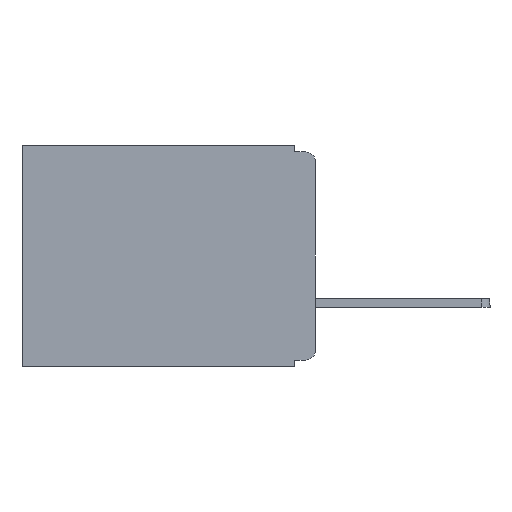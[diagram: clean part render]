
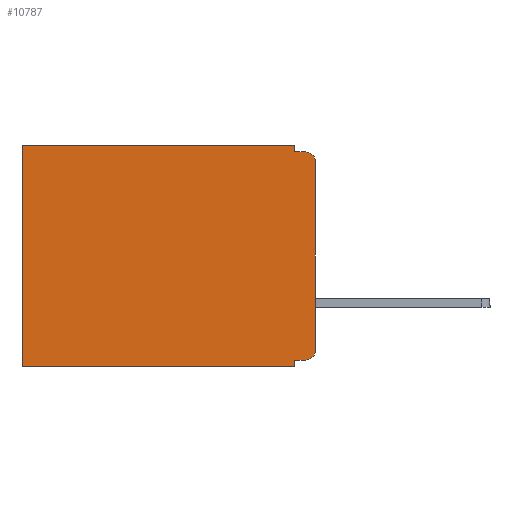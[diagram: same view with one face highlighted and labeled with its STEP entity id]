
A CAD part, left-side view. The second image highlights one B-rep face of the part: STEP entity #10787.
In plain terms, the highlighted planar face has unit normal (-1, 0, 0).
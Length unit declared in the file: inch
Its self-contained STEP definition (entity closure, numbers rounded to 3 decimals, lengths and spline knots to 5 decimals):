
#88 = LINE ( 'NONE', #7431, #16410 ) ;
#299 = CIRCLE ( 'NONE', #828, 0.015 ) ;
#390 = DIRECTION ( 'NONE',  ( 0., 0., -1. ) ) ;
#621 = EDGE_CURVE ( 'NONE', #9456, #8271, #6126, .T. ) ;
#828 = AXIS2_PLACEMENT_3D ( 'NONE', #17038, #7433, #18661 ) ;
#851 = EDGE_CURVE ( 'NONE', #11710, #12561, #5374, .T. ) ;
#950 = DIRECTION ( 'NONE',  ( 0., -1., 0. ) ) ;
#1039 = LINE ( 'NONE', #16659, #19556 ) ;
#1273 = CARTESIAN_POINT ( 'NONE',  ( 0.3, 0.031, -0.33 ) ) ;
#1538 = CIRCLE ( 'NONE', #13195, 0.015 ) ;
#1649 = EDGE_CURVE ( 'NONE', #15379, #8201, #2209, .T. ) ;
#2209 = LINE ( 'NONE', #11035, #15659 ) ;
#2233 = DIRECTION ( 'NONE',  ( 0., 0., -1. ) ) ;
#2253 = VECTOR ( 'NONE', #6494, 39.37008 ) ;
#2718 = CARTESIAN_POINT ( 'NONE',  ( 0.3, 0., -0.305 ) ) ;
#3698 = CARTESIAN_POINT ( 'NONE',  ( 0.3, 0.031, 0. ) ) ;
#3895 = ORIENTED_EDGE ( 'NONE', *, *, #20983, .F. ) ;
#4045 = ORIENTED_EDGE ( 'NONE', *, *, #851, .F. ) ;
#4522 = CARTESIAN_POINT ( 'NONE',  ( 0.3, 0., -0.33 ) ) ;
#4818 = CARTESIAN_POINT ( 'NONE',  ( 0.3, 0.015, -0.305 ) ) ;
#4846 = ORIENTED_EDGE ( 'NONE', *, *, #1649, .T. ) ;
#5374 = LINE ( 'NONE', #1273, #17690 ) ;
#5652 = LINE ( 'NONE', #4522, #13681 ) ;
#6126 = LINE ( 'NONE', #18607, #14677 ) ;
#6450 = EDGE_CURVE ( 'NONE', #10704, #15379, #88, .T. ) ;
#6462 = DIRECTION ( 'NONE',  ( 0., 0., -1. ) ) ;
#6494 = DIRECTION ( 'NONE',  ( 0., 1., 0. ) ) ;
#6562 = CARTESIAN_POINT ( 'NONE',  ( 0.3, 0., -0.32 ) ) ;
#7431 = CARTESIAN_POINT ( 'NONE',  ( 0.3, 0., 0. ) ) ;
#7433 = DIRECTION ( 'NONE',  ( -1., 0., 0. ) ) ;
#8042 = VERTEX_POINT ( 'NONE', #19347 ) ;
#8201 = VERTEX_POINT ( 'NONE', #16296 ) ;
#8271 = VERTEX_POINT ( 'NONE', #10420 ) ;
#8680 = EDGE_CURVE ( 'NONE', #20669, #17223, #1538, .T. ) ;
#8954 = ORIENTED_EDGE ( 'NONE', *, *, #20489, .F. ) ;
#9442 = DIRECTION ( 'NONE',  ( 0., 0., -1. ) ) ;
#9456 = VERTEX_POINT ( 'NONE', #11789 ) ;
#9977 = DIRECTION ( 'NONE',  ( 0., 0., -1. ) ) ;
#10138 = EDGE_CURVE ( 'NONE', #12561, #8201, #1039, .T. ) ;
#10391 = CARTESIAN_POINT ( 'NONE',  ( 0.3, 0., -0.33 ) ) ;
#10420 = CARTESIAN_POINT ( 'NONE',  ( 0.3, 0.015, -0.01 ) ) ;
#10456 = LINE ( 'NONE', #6562, #2253 ) ;
#10574 = CARTESIAN_POINT ( 'NONE',  ( 0.3, 0.437, 0. ) ) ;
#10639 = EDGE_CURVE ( 'NONE', #10704, #9456, #19055, .T. ) ;
#10704 = VERTEX_POINT ( 'NONE', #3698 ) ;
#10787 = ADVANCED_FACE ( 'NONE', ( #15529 ), #19952, .F. ) ;
#11035 = CARTESIAN_POINT ( 'NONE',  ( 0.3, 0.437, -0.33 ) ) ;
#11106 = DIRECTION ( 'NONE',  ( 0., 0., -1. ) ) ;
#11425 = DIRECTION ( 'NONE',  ( 0., 1., 0. ) ) ;
#11710 = VERTEX_POINT ( 'NONE', #20813 ) ;
#11789 = CARTESIAN_POINT ( 'NONE',  ( 0.3, 0.031, -0.01 ) ) ;
#12016 = DIRECTION ( 'NONE',  ( 1., 0., 0. ) ) ;
#12436 = AXIS2_PLACEMENT_3D ( 'NONE', #10391, #12016, #2233 ) ;
#12561 = VERTEX_POINT ( 'NONE', #19966 ) ;
#12746 = ORIENTED_EDGE ( 'NONE', *, *, #10639, .F. ) ;
#13195 = AXIS2_PLACEMENT_3D ( 'NONE', #4818, #16075, #6462 ) ;
#13681 = VECTOR ( 'NONE', #9442, 39.37008 ) ;
#14677 = VECTOR ( 'NONE', #950, 39.37008 ) ;
#14786 = EDGE_CURVE ( 'NONE', #8042, #8271, #299, .T. ) ;
#14794 = VECTOR ( 'NONE', #9977, 39.37008 ) ;
#14969 = CARTESIAN_POINT ( 'NONE',  ( 0.3, 0.015, -0.32 ) ) ;
#15168 = ORIENTED_EDGE ( 'NONE', *, *, #10138, .F. ) ;
#15379 = VERTEX_POINT ( 'NONE', #10574 ) ;
#15427 = ORIENTED_EDGE ( 'NONE', *, *, #6450, .T. ) ;
#15529 = FACE_OUTER_BOUND ( 'NONE', #20500, .T. ) ;
#15659 = VECTOR ( 'NONE', #390, 39.37008 ) ;
#16075 = DIRECTION ( 'NONE',  ( -1., 0., 0. ) ) ;
#16296 = CARTESIAN_POINT ( 'NONE',  ( 0.3, 0.437, -0.33 ) ) ;
#16410 = VECTOR ( 'NONE', #11425, 39.37008 ) ;
#16583 = DIRECTION ( 'NONE',  ( 0., 1., 0. ) ) ;
#16659 = CARTESIAN_POINT ( 'NONE',  ( 0.3, 0., -0.33 ) ) ;
#17038 = CARTESIAN_POINT ( 'NONE',  ( 0.3, 0.015, -0.025 ) ) ;
#17223 = VERTEX_POINT ( 'NONE', #2718 ) ;
#17690 = VECTOR ( 'NONE', #11106, 39.37008 ) ;
#17968 = ORIENTED_EDGE ( 'NONE', *, *, #621, .F. ) ;
#18572 = ORIENTED_EDGE ( 'NONE', *, *, #8680, .T. ) ;
#18607 = CARTESIAN_POINT ( 'NONE',  ( 0.3, 0., -0.01 ) ) ;
#18661 = DIRECTION ( 'NONE',  ( 0., 0., -1. ) ) ;
#19055 = LINE ( 'NONE', #19552, #14794 ) ;
#19347 = CARTESIAN_POINT ( 'NONE',  ( 0.3, 0., -0.025 ) ) ;
#19552 = CARTESIAN_POINT ( 'NONE',  ( 0.3, 0.031, 0. ) ) ;
#19556 = VECTOR ( 'NONE', #16583, 39.37008 ) ;
#19952 = PLANE ( 'NONE',  #12436 ) ;
#19966 = CARTESIAN_POINT ( 'NONE',  ( 0.3, 0.031, -0.33 ) ) ;
#20489 = EDGE_CURVE ( 'NONE', #20669, #11710, #10456, .T. ) ;
#20500 = EDGE_LOOP ( 'NONE', ( #3895, #20739, #17968, #12746, #15427, #4846, #15168, #4045, #8954, #18572 ) ) ;
#20669 = VERTEX_POINT ( 'NONE', #14969 ) ;
#20739 = ORIENTED_EDGE ( 'NONE', *, *, #14786, .T. ) ;
#20813 = CARTESIAN_POINT ( 'NONE',  ( 0.3, 0.031, -0.32 ) ) ;
#20983 = EDGE_CURVE ( 'NONE', #8042, #17223, #5652, .T. ) ;
